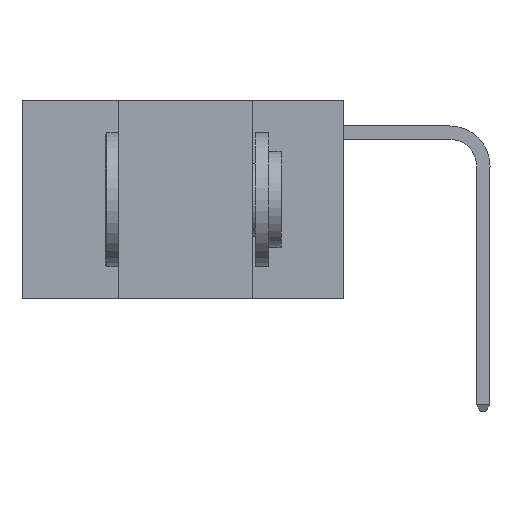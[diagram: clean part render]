
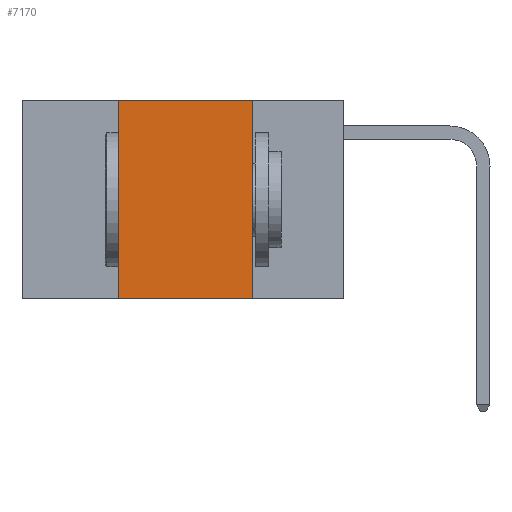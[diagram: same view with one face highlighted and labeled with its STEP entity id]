
A CAD part, left-side view. The second image highlights one B-rep face of the part: STEP entity #7170.
In plain terms, the highlighted planar face has unit normal (-1, 0, 0).
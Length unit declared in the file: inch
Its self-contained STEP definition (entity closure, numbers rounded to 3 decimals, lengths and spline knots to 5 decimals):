
#561 = VECTOR ( 'NONE', #6779, 39.37008 ) ;
#731 = ORIENTED_EDGE ( 'NONE', *, *, #1507, .T. ) ;
#982 = AXIS2_PLACEMENT_3D ( 'NONE', #2994, #4144, #12299 ) ;
#1507 = EDGE_CURVE ( 'NONE', #5807, #8856, #14181, .T. ) ;
#1527 = VERTEX_POINT ( 'NONE', #2618 ) ;
#1773 = PLANE ( 'NONE',  #982 ) ;
#2618 = CARTESIAN_POINT ( 'NONE',  ( 0., 0.17, 0. ) ) ;
#2681 = LINE ( 'NONE', #3673, #6142 ) ;
#2853 = DIRECTION ( 'NONE',  ( 0., -1., 0. ) ) ;
#2994 = CARTESIAN_POINT ( 'NONE',  ( 0., 0.6, 0. ) ) ;
#3185 = CARTESIAN_POINT ( 'NONE',  ( 0., 0.42, 0. ) ) ;
#3564 = ORIENTED_EDGE ( 'NONE', *, *, #12660, .F. ) ;
#3673 = CARTESIAN_POINT ( 'NONE',  ( 0., 0.6, 0. ) ) ;
#3749 = FACE_OUTER_BOUND ( 'NONE', #13874, .T. ) ;
#3840 = VECTOR ( 'NONE', #10595, 39.37008 ) ;
#4144 = DIRECTION ( 'NONE',  ( 1., 0., 0. ) ) ;
#4565 = VERTEX_POINT ( 'NONE', #3185 ) ;
#4932 = VECTOR ( 'NONE', #2853, 39.37008 ) ;
#5601 = CARTESIAN_POINT ( 'NONE',  ( 0., 0.17, 0. ) ) ;
#5807 = VERTEX_POINT ( 'NONE', #13252 ) ;
#6142 = VECTOR ( 'NONE', #14012, 39.37008 ) ;
#6779 = DIRECTION ( 'NONE',  ( 0., 0., -1. ) ) ;
#7170 = ADVANCED_FACE ( 'NONE', ( #3749 ), #1773, .F. ) ;
#8856 = VERTEX_POINT ( 'NONE', #9763 ) ;
#9398 = ORIENTED_EDGE ( 'NONE', *, *, #13149, .F. ) ;
#9449 = CARTESIAN_POINT ( 'NONE',  ( 0., 0.42, 0. ) ) ;
#9756 = ORIENTED_EDGE ( 'NONE', *, *, #10505, .F. ) ;
#9763 = CARTESIAN_POINT ( 'NONE',  ( 0., 0.17, -0.37 ) ) ;
#9970 = LINE ( 'NONE', #5601, #561 ) ;
#10046 = LINE ( 'NONE', #9449, #3840 ) ;
#10505 = EDGE_CURVE ( 'NONE', #5807, #4565, #10046, .T. ) ;
#10595 = DIRECTION ( 'NONE',  ( 0., 0., 1. ) ) ;
#12299 = DIRECTION ( 'NONE',  ( 0., 0., -1. ) ) ;
#12660 = EDGE_CURVE ( 'NONE', #4565, #1527, #2681, .T. ) ;
#13149 = EDGE_CURVE ( 'NONE', #1527, #8856, #9970, .T. ) ;
#13252 = CARTESIAN_POINT ( 'NONE',  ( 0., 0.42, -0.37 ) ) ;
#13874 = EDGE_LOOP ( 'NONE', ( #9398, #3564, #9756, #731 ) ) ;
#14012 = DIRECTION ( 'NONE',  ( 0., -1., 0. ) ) ;
#14181 = LINE ( 'NONE', #15131, #4932 ) ;
#15131 = CARTESIAN_POINT ( 'NONE',  ( 0., 0.6, -0.37 ) ) ;
